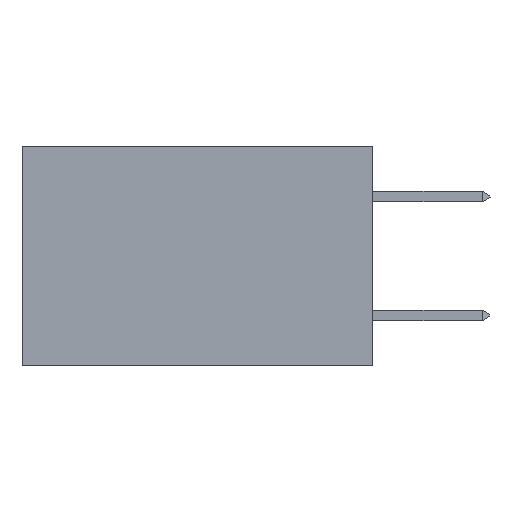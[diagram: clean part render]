
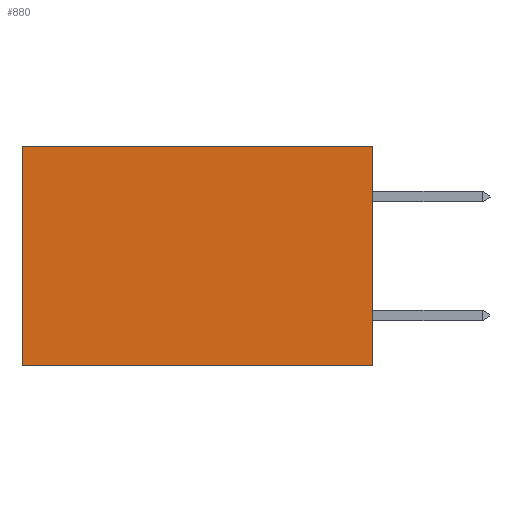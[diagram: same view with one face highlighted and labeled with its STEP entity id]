
A CAD part, left-side view. The second image highlights one B-rep face of the part: STEP entity #880.
In plain terms, the highlighted planar face has unit normal (-1, 0, 0).
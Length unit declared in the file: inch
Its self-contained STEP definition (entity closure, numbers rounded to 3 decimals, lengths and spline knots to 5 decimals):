
#48 = ORIENTED_EDGE ( 'NONE', *, *, #14970, .F. ) ;
#326 = FACE_OUTER_BOUND ( 'NONE', #3493, .T. ) ;
#880 = ADVANCED_FACE ( 'NONE', ( #326 ), #21360, .F. ) ;
#2780 = CARTESIAN_POINT ( 'NONE',  ( 0.277, 0., -0.37 ) ) ;
#3493 = EDGE_LOOP ( 'NONE', ( #25165, #15587, #48, #8862 ) ) ;
#3687 = EDGE_CURVE ( 'NONE', #7851, #24386, #25462, .T. ) ;
#4120 = LINE ( 'NONE', #2780, #8556 ) ;
#6548 = CARTESIAN_POINT ( 'NONE',  ( 0.277, 0.59, 0. ) ) ;
#6959 = VERTEX_POINT ( 'NONE', #16169 ) ;
#7398 = VECTOR ( 'NONE', #8185, 39.37008 ) ;
#7851 = VERTEX_POINT ( 'NONE', #8689 ) ;
#8185 = DIRECTION ( 'NONE',  ( 0., 0., -1. ) ) ;
#8269 = DIRECTION ( 'NONE',  ( 1., 0., 0. ) ) ;
#8556 = VECTOR ( 'NONE', #18042, 39.37008 ) ;
#8689 = CARTESIAN_POINT ( 'NONE',  ( 0.277, 0., 0. ) ) ;
#8862 = ORIENTED_EDGE ( 'NONE', *, *, #3687, .T. ) ;
#9185 = EDGE_CURVE ( 'NONE', #17794, #6959, #4120, .T. ) ;
#9711 = VECTOR ( 'NONE', #13620, 39.37008 ) ;
#11523 = CARTESIAN_POINT ( 'NONE',  ( 0.277, 0., 0. ) ) ;
#11674 = CARTESIAN_POINT ( 'NONE',  ( 0.277, 0., -0.37 ) ) ;
#13155 = VECTOR ( 'NONE', #18108, 39.37008 ) ;
#13620 = DIRECTION ( 'NONE',  ( 0., 0., -1. ) ) ;
#14970 = EDGE_CURVE ( 'NONE', #7851, #17794, #22021, .T. ) ;
#15587 = ORIENTED_EDGE ( 'NONE', *, *, #9185, .F. ) ;
#16169 = CARTESIAN_POINT ( 'NONE',  ( 0.277, 0.59, -0.37 ) ) ;
#17794 = VERTEX_POINT ( 'NONE', #11674 ) ;
#18042 = DIRECTION ( 'NONE',  ( 0., 1., 0. ) ) ;
#18108 = DIRECTION ( 'NONE',  ( 0., 1., 0. ) ) ;
#19007 = LINE ( 'NONE', #21270, #7398 ) ;
#19146 = CARTESIAN_POINT ( 'NONE',  ( 0.277, 0., -0.37 ) ) ;
#20100 = EDGE_CURVE ( 'NONE', #24386, #6959, #19007, .T. ) ;
#21270 = CARTESIAN_POINT ( 'NONE',  ( 0.277, 0.59, -0.37 ) ) ;
#21360 = PLANE ( 'NONE',  #22807 ) ;
#22021 = LINE ( 'NONE', #24505, #9711 ) ;
#22807 = AXIS2_PLACEMENT_3D ( 'NONE', #19146, #8269, #23550 ) ;
#23550 = DIRECTION ( 'NONE',  ( 0., 0., -1. ) ) ;
#24386 = VERTEX_POINT ( 'NONE', #6548 ) ;
#24505 = CARTESIAN_POINT ( 'NONE',  ( 0.277, 0., -0.37 ) ) ;
#25165 = ORIENTED_EDGE ( 'NONE', *, *, #20100, .T. ) ;
#25462 = LINE ( 'NONE', #11523, #13155 ) ;
